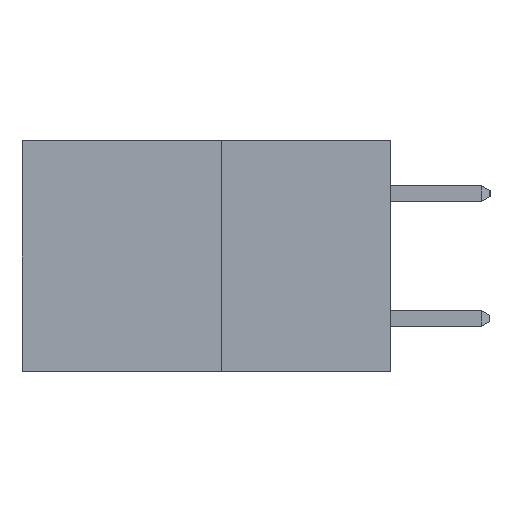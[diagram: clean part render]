
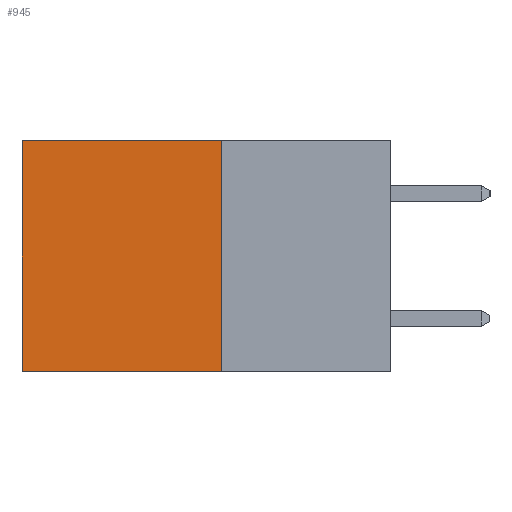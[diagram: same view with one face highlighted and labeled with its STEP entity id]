
A CAD part, left-side view. The second image highlights one B-rep face of the part: STEP entity #945.
In plain terms, the highlighted planar face has unit normal (-1, 0, 0).
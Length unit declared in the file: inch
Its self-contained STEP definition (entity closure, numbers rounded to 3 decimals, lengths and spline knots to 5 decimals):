
#801 = DIRECTION ( 'NONE',  ( 0., 1., 0. ) ) ;
#945 = ADVANCED_FACE ( 'NONE', ( #10204 ), #9569, .F. ) ;
#1997 = VERTEX_POINT ( 'NONE', #8837 ) ;
#2030 = EDGE_LOOP ( 'NONE', ( #10824, #4507, #6763, #11058 ) ) ;
#2220 = VECTOR ( 'NONE', #801, 39.37008 ) ;
#2410 = CARTESIAN_POINT ( 'NONE',  ( 0.277, 0.59, -0.37 ) ) ;
#2609 = LINE ( 'NONE', #10007, #4888 ) ;
#2685 = CARTESIAN_POINT ( 'NONE',  ( 0.277, 0.27, -0.37 ) ) ;
#2941 = EDGE_CURVE ( 'NONE', #9714, #6091, #8187, .T. ) ;
#3716 = VECTOR ( 'NONE', #9997, 39.37008 ) ;
#3940 = AXIS2_PLACEMENT_3D ( 'NONE', #2685, #5079, #5040 ) ;
#4047 = EDGE_CURVE ( 'NONE', #1997, #9714, #6770, .T. ) ;
#4507 = ORIENTED_EDGE ( 'NONE', *, *, #4637, .F. ) ;
#4637 = EDGE_CURVE ( 'NONE', #10058, #6091, #2609, .T. ) ;
#4888 = VECTOR ( 'NONE', #10760, 39.37008 ) ;
#5040 = DIRECTION ( 'NONE',  ( 0., 0., -1. ) ) ;
#5060 = CARTESIAN_POINT ( 'NONE',  ( 0.277, 0.59, 0. ) ) ;
#5079 = DIRECTION ( 'NONE',  ( 1., 0., 0. ) ) ;
#5436 = CARTESIAN_POINT ( 'NONE',  ( 0.277, 0.27, -0.37 ) ) ;
#6091 = VERTEX_POINT ( 'NONE', #6701 ) ;
#6701 = CARTESIAN_POINT ( 'NONE',  ( 0.277, 0.59, -0.37 ) ) ;
#6763 = ORIENTED_EDGE ( 'NONE', *, *, #7434, .F. ) ;
#6770 = LINE ( 'NONE', #11025, #2220 ) ;
#7026 = CARTESIAN_POINT ( 'NONE',  ( 0.277, 0.27, -0.37 ) ) ;
#7434 = EDGE_CURVE ( 'NONE', #1997, #10058, #10298, .T. ) ;
#7933 = DIRECTION ( 'NONE',  ( 0., 0., -1. ) ) ;
#8100 = VECTOR ( 'NONE', #7933, 39.37008 ) ;
#8187 = LINE ( 'NONE', #2410, #3716 ) ;
#8837 = CARTESIAN_POINT ( 'NONE',  ( 0.277, 0.27, 0. ) ) ;
#9569 = PLANE ( 'NONE',  #3940 ) ;
#9714 = VERTEX_POINT ( 'NONE', #5060 ) ;
#9997 = DIRECTION ( 'NONE',  ( 0., 0., -1. ) ) ;
#10007 = CARTESIAN_POINT ( 'NONE',  ( 0.277, 0.27, -0.37 ) ) ;
#10058 = VERTEX_POINT ( 'NONE', #7026 ) ;
#10204 = FACE_OUTER_BOUND ( 'NONE', #2030, .T. ) ;
#10298 = LINE ( 'NONE', #5436, #8100 ) ;
#10760 = DIRECTION ( 'NONE',  ( 0., 1., 0. ) ) ;
#10824 = ORIENTED_EDGE ( 'NONE', *, *, #2941, .T. ) ;
#11025 = CARTESIAN_POINT ( 'NONE',  ( 0.277, 0.27, 0. ) ) ;
#11058 = ORIENTED_EDGE ( 'NONE', *, *, #4047, .T. ) ;
